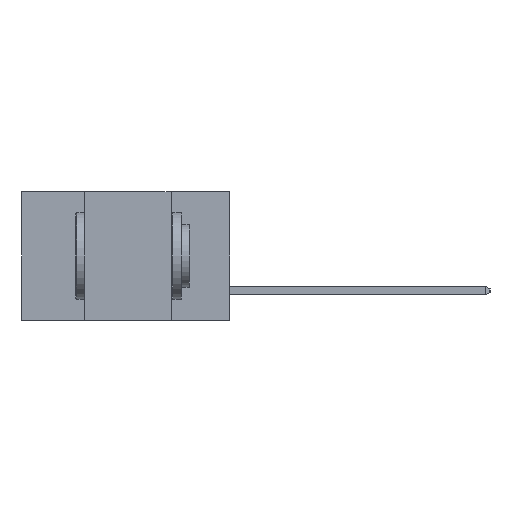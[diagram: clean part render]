
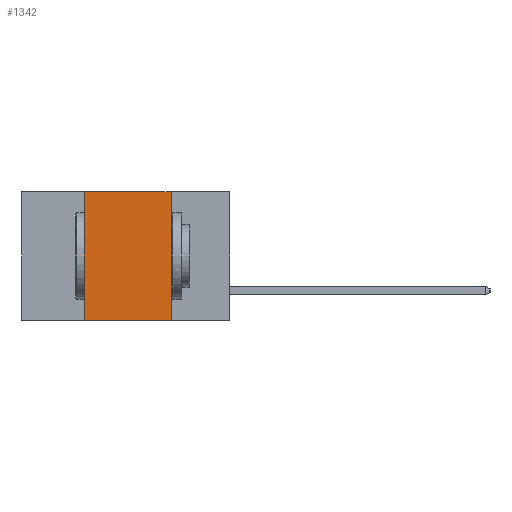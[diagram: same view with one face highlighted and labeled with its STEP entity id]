
A CAD part, left-side view. The second image highlights one B-rep face of the part: STEP entity #1342.
In plain terms, the highlighted planar face has unit normal (-1, 0, 0).
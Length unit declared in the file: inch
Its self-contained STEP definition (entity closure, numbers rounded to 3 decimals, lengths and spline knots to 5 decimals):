
#1342 = ADVANCED_FACE ( 'NONE', ( #4694 ), #13375, .F. ) ;
#1748 = EDGE_LOOP ( 'NONE', ( #12990, #8190, #13273, #3380 ) ) ;
#2899 = CARTESIAN_POINT ( 'NONE',  ( 0., 0.6, -0.37 ) ) ;
#3380 = ORIENTED_EDGE ( 'NONE', *, *, #4069, .T. ) ;
#4069 = EDGE_CURVE ( 'NONE', #10948, #6466, #5010, .T. ) ;
#4661 = CARTESIAN_POINT ( 'NONE',  ( 0., 0.42, -0.37 ) ) ;
#4694 = FACE_OUTER_BOUND ( 'NONE', #1748, .T. ) ;
#4756 = EDGE_CURVE ( 'NONE', #10948, #6848, #11378, .T. ) ;
#4816 = VECTOR ( 'NONE', #5590, 39.37008 ) ;
#5010 = LINE ( 'NONE', #2899, #12266 ) ;
#5120 = LINE ( 'NONE', #11404, #10739 ) ;
#5396 = CARTESIAN_POINT ( 'NONE',  ( 0., 0.42, 0. ) ) ;
#5445 = EDGE_CURVE ( 'NONE', #6848, #8150, #10475, .T. ) ;
#5458 = DIRECTION ( 'NONE',  ( 0., 0., -1. ) ) ;
#5590 = DIRECTION ( 'NONE',  ( 0., -1., 0. ) ) ;
#6116 = EDGE_CURVE ( 'NONE', #8150, #6466, #5120, .T. ) ;
#6466 = VERTEX_POINT ( 'NONE', #12659 ) ;
#6848 = VERTEX_POINT ( 'NONE', #5396 ) ;
#6882 = DIRECTION ( 'NONE',  ( 0., 0., 1. ) ) ;
#8150 = VERTEX_POINT ( 'NONE', #11286 ) ;
#8190 = ORIENTED_EDGE ( 'NONE', *, *, #5445, .F. ) ;
#9032 = DIRECTION ( 'NONE',  ( 0., -1., 0. ) ) ;
#9603 = CARTESIAN_POINT ( 'NONE',  ( 0., 0.6, 0. ) ) ;
#9783 = AXIS2_PLACEMENT_3D ( 'NONE', #13173, #12592, #12578 ) ;
#10475 = LINE ( 'NONE', #9603, #4816 ) ;
#10739 = VECTOR ( 'NONE', #5458, 39.37008 ) ;
#10948 = VERTEX_POINT ( 'NONE', #4661 ) ;
#11286 = CARTESIAN_POINT ( 'NONE',  ( 0., 0.17, 0. ) ) ;
#11378 = LINE ( 'NONE', #12731, #13283 ) ;
#11404 = CARTESIAN_POINT ( 'NONE',  ( 0., 0.17, -0.37 ) ) ;
#12266 = VECTOR ( 'NONE', #9032, 39.37008 ) ;
#12578 = DIRECTION ( 'NONE',  ( 0., 0., -1. ) ) ;
#12592 = DIRECTION ( 'NONE',  ( 1., 0., 0. ) ) ;
#12659 = CARTESIAN_POINT ( 'NONE',  ( 0., 0.17, -0.37 ) ) ;
#12731 = CARTESIAN_POINT ( 'NONE',  ( 0., 0.42, -0.37 ) ) ;
#12990 = ORIENTED_EDGE ( 'NONE', *, *, #6116, .F. ) ;
#13173 = CARTESIAN_POINT ( 'NONE',  ( 0., 0.6, 0. ) ) ;
#13273 = ORIENTED_EDGE ( 'NONE', *, *, #4756, .F. ) ;
#13283 = VECTOR ( 'NONE', #6882, 39.37008 ) ;
#13375 = PLANE ( 'NONE',  #9783 ) ;
